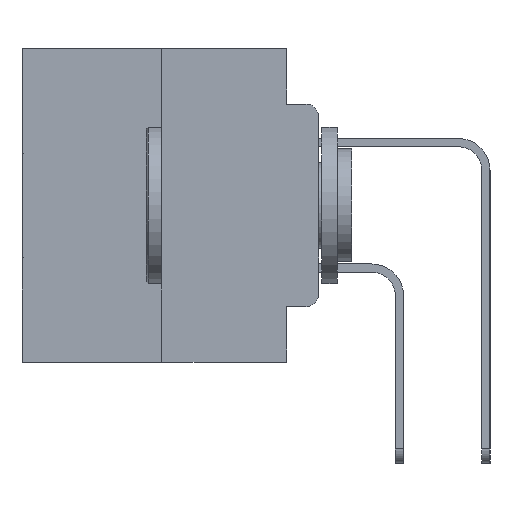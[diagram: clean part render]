
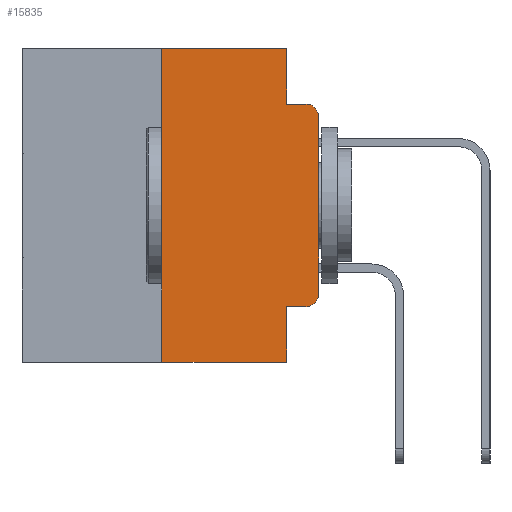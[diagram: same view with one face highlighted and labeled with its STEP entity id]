
A CAD part, left-side view. The second image highlights one B-rep face of the part: STEP entity #15835.
In plain terms, the highlighted planar face has unit normal (-1, 0, 0).
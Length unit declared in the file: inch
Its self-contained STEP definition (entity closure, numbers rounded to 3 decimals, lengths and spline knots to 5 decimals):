
#1182 = DIRECTION ( 'NONE',  ( 0., -1., 0. ) ) ;
#1643 = VERTEX_POINT ( 'NONE', #1982 ) ;
#1982 = CARTESIAN_POINT ( 'NONE',  ( 0., 0., -0.1085 ) ) ;
#3830 = CARTESIAN_POINT ( 'NONE',  ( 0., 0.473, 0. ) ) ;
#3840 = VERTEX_POINT ( 'NONE', #16285 ) ;
#4189 = CARTESIAN_POINT ( 'NONE',  ( 0., 0.051, 0. ) ) ;
#4617 = EDGE_LOOP ( 'NONE', ( #12949, #13064, #14715, #14884, #15220, #16066, #16611, #17186, #17221, #17253 ) ) ;
#4708 = EDGE_CURVE ( 'NONE', #3840, #1643, #11417, .T. ) ;
#4977 = DIRECTION ( 'NONE',  ( -1., 0., 0. ) ) ;
#5016 = DIRECTION ( 'NONE',  ( 0., 0., -1. ) ) ;
#5221 = LINE ( 'NONE', #13362, #11698 ) ;
#5650 = EDGE_CURVE ( 'NONE', #27184, #3840, #28723, .T. ) ;
#6474 = CARTESIAN_POINT ( 'NONE',  ( 0., 0.02, -0.1085 ) ) ;
#6928 = DIRECTION ( 'NONE',  ( 0., 0., 1. ) ) ;
#7619 = LINE ( 'NONE', #3830, #25871 ) ;
#7955 = CARTESIAN_POINT ( 'NONE',  ( 0., 0.051, -0.0885 ) ) ;
#8099 = VERTEX_POINT ( 'NONE', #29438 ) ;
#8354 = VECTOR ( 'NONE', #29319, 39.37008 ) ;
#8579 = CARTESIAN_POINT ( 'NONE',  ( 0., 0.02, -0.3915 ) ) ;
#8860 = VERTEX_POINT ( 'NONE', #20867 ) ;
#8925 = DIRECTION ( 'NONE',  ( 0., 0., -1. ) ) ;
#9009 = LINE ( 'NONE', #14735, #21699 ) ;
#9170 = PLANE ( 'NONE',  #17616 ) ;
#9231 = EDGE_CURVE ( 'NONE', #8099, #27184, #25994, .T. ) ;
#10562 = VERTEX_POINT ( 'NONE', #18274 ) ;
#11250 = EDGE_CURVE ( 'NONE', #1643, #13878, #22177, .T. ) ;
#11417 = LINE ( 'NONE', #21866, #17035 ) ;
#11586 = CARTESIAN_POINT ( 'NONE',  ( 0., 0.473, 0. ) ) ;
#11698 = VECTOR ( 'NONE', #15651, 39.37008 ) ;
#12949 = ORIENTED_EDGE ( 'NONE', *, *, #4708, .T. ) ;
#13064 = ORIENTED_EDGE ( 'NONE', *, *, #11250, .T. ) ;
#13307 = VERTEX_POINT ( 'NONE', #21899 ) ;
#13362 = CARTESIAN_POINT ( 'NONE',  ( 0., 0.473, -0.5 ) ) ;
#13402 = VECTOR ( 'NONE', #15002, 39.37008 ) ;
#13878 = VERTEX_POINT ( 'NONE', #14369 ) ;
#13974 = DIRECTION ( 'NONE',  ( 1., 0., 0. ) ) ;
#14369 = CARTESIAN_POINT ( 'NONE',  ( 0., 0.02, -0.0885 ) ) ;
#14551 = CARTESIAN_POINT ( 'NONE',  ( 0., 0.25, 0. ) ) ;
#14715 = ORIENTED_EDGE ( 'NONE', *, *, #23554, .F. ) ;
#14735 = CARTESIAN_POINT ( 'NONE',  ( 0., 0.051, 0. ) ) ;
#14884 = ORIENTED_EDGE ( 'NONE', *, *, #27271, .F. ) ;
#15002 = DIRECTION ( 'NONE',  ( 0., -1., 0. ) ) ;
#15079 = DIRECTION ( 'NONE',  ( 0., -1., 0. ) ) ;
#15220 = ORIENTED_EDGE ( 'NONE', *, *, #16916, .F. ) ;
#15651 = DIRECTION ( 'NONE',  ( 0., -1., 0. ) ) ;
#15835 = ADVANCED_FACE ( 'NONE', ( #15887 ), #9170, .F. ) ;
#15887 = FACE_OUTER_BOUND ( 'NONE', #4617, .T. ) ;
#16066 = ORIENTED_EDGE ( 'NONE', *, *, #27696, .F. ) ;
#16285 = CARTESIAN_POINT ( 'NONE',  ( 0., 0., -0.3915 ) ) ;
#16611 = ORIENTED_EDGE ( 'NONE', *, *, #17845, .T. ) ;
#16627 = CARTESIAN_POINT ( 'NONE',  ( 0., 0.051, -0.5 ) ) ;
#16916 = EDGE_CURVE ( 'NONE', #10562, #19865, #7619, .T. ) ;
#17035 = VECTOR ( 'NONE', #6928, 39.37008 ) ;
#17148 = DIRECTION ( 'NONE',  ( 0., 0., -1. ) ) ;
#17186 = ORIENTED_EDGE ( 'NONE', *, *, #26018, .F. ) ;
#17221 = ORIENTED_EDGE ( 'NONE', *, *, #9231, .T. ) ;
#17253 = ORIENTED_EDGE ( 'NONE', *, *, #5650, .T. ) ;
#17616 = AXIS2_PLACEMENT_3D ( 'NONE', #11586, #13974, #30381 ) ;
#17845 = EDGE_CURVE ( 'NONE', #8860, #27141, #5221, .T. ) ;
#18274 = CARTESIAN_POINT ( 'NONE',  ( 0., 0.25, 0. ) ) ;
#18497 = AXIS2_PLACEMENT_3D ( 'NONE', #6474, #23214, #8925 ) ;
#19865 = VERTEX_POINT ( 'NONE', #4189 ) ;
#20867 = CARTESIAN_POINT ( 'NONE',  ( 0., 0.25, -0.5 ) ) ;
#20943 = VECTOR ( 'NONE', #30909, 39.37008 ) ;
#21699 = VECTOR ( 'NONE', #17148, 39.37008 ) ;
#21866 = CARTESIAN_POINT ( 'NONE',  ( 0., 0., 0. ) ) ;
#21895 = VECTOR ( 'NONE', #15079, 39.37008 ) ;
#21899 = CARTESIAN_POINT ( 'NONE',  ( 0., 0.051, -0.0885 ) ) ;
#22177 = CIRCLE ( 'NONE', #18497, 0.02 ) ;
#22181 = CARTESIAN_POINT ( 'NONE',  ( 0., 0.051, -0.4115 ) ) ;
#22635 = LINE ( 'NONE', #7955, #21895 ) ;
#23214 = DIRECTION ( 'NONE',  ( -1., 0., 0. ) ) ;
#23554 = EDGE_CURVE ( 'NONE', #13307, #13878, #22635, .T. ) ;
#23884 = CARTESIAN_POINT ( 'NONE',  ( 0., 0.02, -0.4115 ) ) ;
#25871 = VECTOR ( 'NONE', #1182, 39.37008 ) ;
#25994 = LINE ( 'NONE', #22181, #13402 ) ;
#26018 = EDGE_CURVE ( 'NONE', #8099, #27141, #27296, .T. ) ;
#26443 = LINE ( 'NONE', #14551, #20943 ) ;
#27039 = CARTESIAN_POINT ( 'NONE',  ( 0., 0.051, 0. ) ) ;
#27141 = VERTEX_POINT ( 'NONE', #16627 ) ;
#27184 = VERTEX_POINT ( 'NONE', #23884 ) ;
#27271 = EDGE_CURVE ( 'NONE', #19865, #13307, #9009, .T. ) ;
#27296 = LINE ( 'NONE', #27039, #8354 ) ;
#27696 = EDGE_CURVE ( 'NONE', #8860, #10562, #26443, .T. ) ;
#28038 = AXIS2_PLACEMENT_3D ( 'NONE', #8579, #4977, #5016 ) ;
#28723 = CIRCLE ( 'NONE', #28038, 0.02 ) ;
#29319 = DIRECTION ( 'NONE',  ( 0., 0., -1. ) ) ;
#29438 = CARTESIAN_POINT ( 'NONE',  ( 0., 0.051, -0.4115 ) ) ;
#30381 = DIRECTION ( 'NONE',  ( 0., 0., -1. ) ) ;
#30909 = DIRECTION ( 'NONE',  ( 0., 0., 1. ) ) ;
